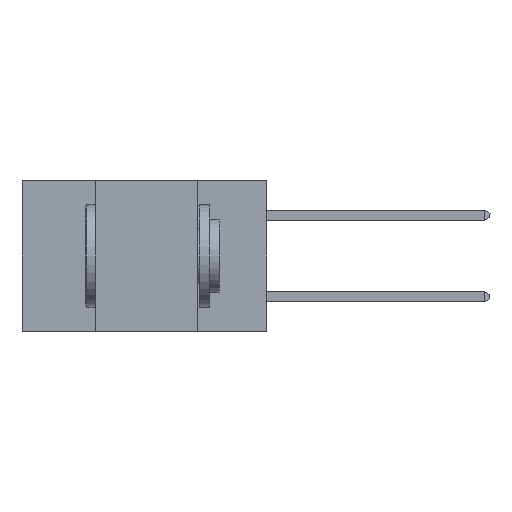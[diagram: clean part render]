
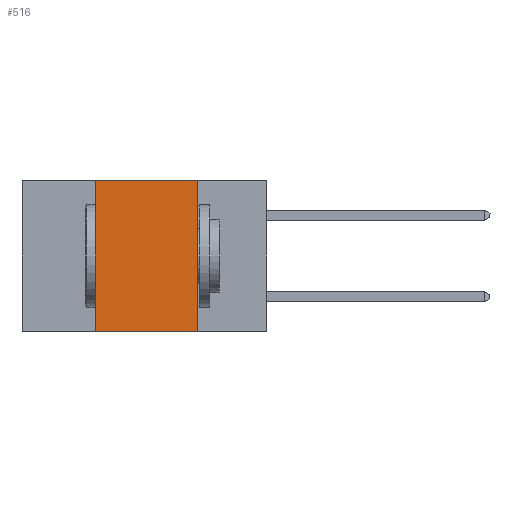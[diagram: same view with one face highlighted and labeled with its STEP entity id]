
A CAD part, left-side view. The second image highlights one B-rep face of the part: STEP entity #516.
In plain terms, the highlighted planar face has unit normal (-1, 0, 0).
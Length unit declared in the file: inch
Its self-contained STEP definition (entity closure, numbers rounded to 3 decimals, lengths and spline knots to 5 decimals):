
#311 = CARTESIAN_POINT ( 'NONE',  ( 0., 0.6, 0. ) ) ;
#516 = ADVANCED_FACE ( 'NONE', ( #12474 ), #1250, .F. ) ;
#623 = DIRECTION ( 'NONE',  ( 1., 0., 0. ) ) ;
#732 = DIRECTION ( 'NONE',  ( 0., 0., -1. ) ) ;
#1228 = CARTESIAN_POINT ( 'NONE',  ( 0., 0.6, 0. ) ) ;
#1250 = PLANE ( 'NONE',  #8931 ) ;
#1552 = DIRECTION ( 'NONE',  ( 0., -1., 0. ) ) ;
#2261 = LINE ( 'NONE', #4611, #12279 ) ;
#3359 = VERTEX_POINT ( 'NONE', #3602 ) ;
#3490 = VECTOR ( 'NONE', #12786, 39.37008 ) ;
#3602 = CARTESIAN_POINT ( 'NONE',  ( 0., 0.42, 0. ) ) ;
#4087 = VERTEX_POINT ( 'NONE', #11291 ) ;
#4611 = CARTESIAN_POINT ( 'NONE',  ( 0., 0.6, -0.37 ) ) ;
#5219 = EDGE_CURVE ( 'NONE', #8616, #4087, #11526, .T. ) ;
#5665 = EDGE_LOOP ( 'NONE', ( #9494, #7541, #12500, #10345 ) ) ;
#5877 = EDGE_CURVE ( 'NONE', #11174, #3359, #12493, .T. ) ;
#6548 = EDGE_CURVE ( 'NONE', #11174, #4087, #2261, .T. ) ;
#6947 = VECTOR ( 'NONE', #10134, 39.37008 ) ;
#7206 = CARTESIAN_POINT ( 'NONE',  ( 0., 0.17, 0. ) ) ;
#7276 = CARTESIAN_POINT ( 'NONE',  ( 0., 0.42, 0. ) ) ;
#7329 = EDGE_CURVE ( 'NONE', #3359, #8616, #10240, .T. ) ;
#7541 = ORIENTED_EDGE ( 'NONE', *, *, #7329, .F. ) ;
#7599 = DIRECTION ( 'NONE',  ( 0., -1., 0. ) ) ;
#8616 = VERTEX_POINT ( 'NONE', #10013 ) ;
#8931 = AXIS2_PLACEMENT_3D ( 'NONE', #1228, #623, #732 ) ;
#9494 = ORIENTED_EDGE ( 'NONE', *, *, #5219, .F. ) ;
#10013 = CARTESIAN_POINT ( 'NONE',  ( 0., 0.17, 0. ) ) ;
#10134 = DIRECTION ( 'NONE',  ( 0., 0., 1. ) ) ;
#10240 = LINE ( 'NONE', #311, #12688 ) ;
#10345 = ORIENTED_EDGE ( 'NONE', *, *, #6548, .T. ) ;
#11174 = VERTEX_POINT ( 'NONE', #11978 ) ;
#11291 = CARTESIAN_POINT ( 'NONE',  ( 0., 0.17, -0.37 ) ) ;
#11526 = LINE ( 'NONE', #7206, #3490 ) ;
#11978 = CARTESIAN_POINT ( 'NONE',  ( 0., 0.42, -0.37 ) ) ;
#12279 = VECTOR ( 'NONE', #7599, 39.37008 ) ;
#12474 = FACE_OUTER_BOUND ( 'NONE', #5665, .T. ) ;
#12493 = LINE ( 'NONE', #7276, #6947 ) ;
#12500 = ORIENTED_EDGE ( 'NONE', *, *, #5877, .F. ) ;
#12688 = VECTOR ( 'NONE', #1552, 39.37008 ) ;
#12786 = DIRECTION ( 'NONE',  ( 0., 0., -1. ) ) ;
